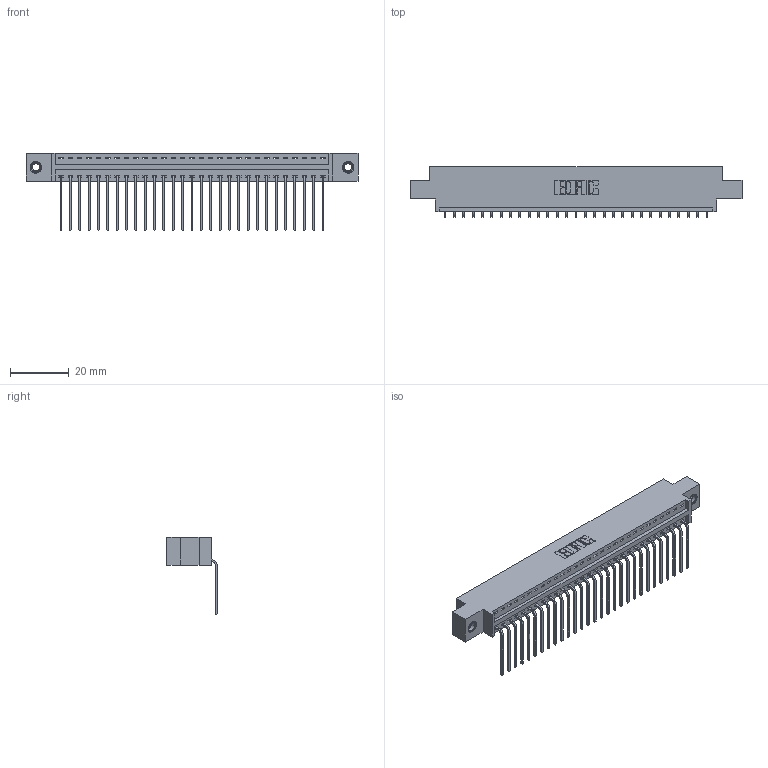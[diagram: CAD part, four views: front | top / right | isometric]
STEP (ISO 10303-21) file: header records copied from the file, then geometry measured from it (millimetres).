
FILE_DESCRIPTION (( 'STEP AP203' ), '1' );
FILE_NAME ('346-029-559-607.STEP', '2022-05-06T15:05:23', ( '' ), ( '' ), 'SwSTEP 2.0', 'SolidWorks 2020', '' );
FILE_SCHEMA (( 'CONFIG_CONTROL_DESIGN' ));
Length unit declared in the file: inch
Products named in the file (4): 346 Part_0.170 Offset - 0.156 Dia-TI; 345-292-001_558 559 Tail - 1; 345-250-001_345-250-005-103; 346-029-559-607
Assembly tree (32 placements, depth 2):
  346-029-559-607
    346 Part_0.170 Offset - 0.156 Dia-TI
    345-292-001_558 559 Tail - 1  x29
    345-250-001_345-250-005-103  x2
Bounding box: 112.65 x 17.08 x 26.16 mm (x, y, z)
Volume: 10621.9 mm3; surface area: 13907.2 mm2
Topology: 32 solids, 32 shells, 1926 faces, 5755 edges, 3790 vertices
Faces by surface type: plane 1330, cylinder 580, cone 12, torus 4
Entity records: 21150 total; most frequent: CARTESIAN_POINT 3614, ORIENTED_EDGE 3570, DIRECTION 3229, EDGE_CURVE 1785, VECTOR 1517, LINE 1517, VERTEX_POINT 1184, AXIS2_PLACEMENT_3D 856
